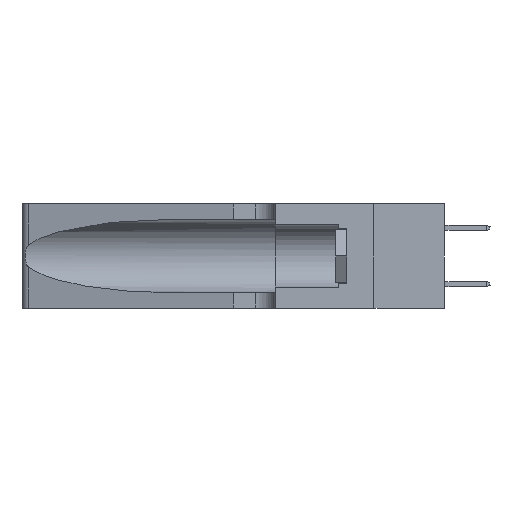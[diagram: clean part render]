
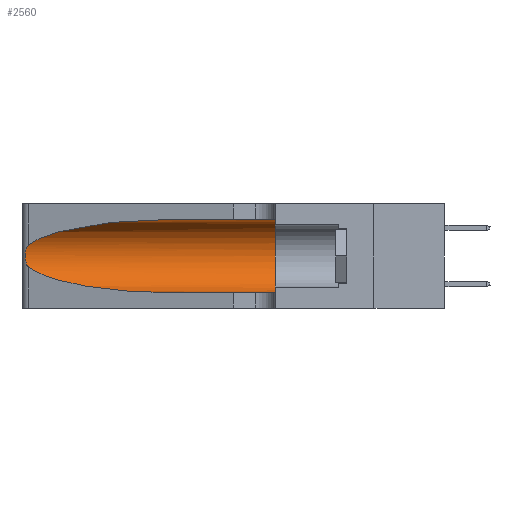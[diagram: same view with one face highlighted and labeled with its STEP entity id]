
A CAD part, left-side view. The second image highlights one B-rep face of the part: STEP entity #2560.
In plain terms, the highlighted cylindrical face has radius 3.308 mm (diameter 6.617 mm), a partial arc.
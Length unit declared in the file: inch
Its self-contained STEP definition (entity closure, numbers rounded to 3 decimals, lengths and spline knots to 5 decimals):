
#1256 = EDGE_CURVE ( 'NONE', #25489, #33092, #20155, .T. ) ;
#1306 = CARTESIAN_POINT ( 'NONE',  ( 0.1305, 0.35, 0.185 ) ) ;
#1328 = DIRECTION ( 'NONE',  ( 0., -1., 0. ) ) ;
#1472 = DIRECTION ( 'NONE',  ( 0., 0., -1. ) ) ;
#2560 = ADVANCED_FACE ( 'NONE', ( #18975 ), #17908, .F. ) ;
#2802 = CARTESIAN_POINT ( 'NONE',  ( 0.25639, 1.23186, 0.15144 ) ) ;
#3285 = VERTEX_POINT ( 'NONE', #24985 ) ;
#3725 = VERTEX_POINT ( 'NONE', #6746 ) ;
#4395 = EDGE_CURVE ( 'NONE', #14317, #3725, #28482, .T. ) ;
#4875 = CARTESIAN_POINT ( 'NONE',  ( 0.2373, 1.15595, 0.28018 ) ) ;
#5112 = ORIENTED_EDGE ( 'NONE', *, *, #26190, .T. ) ;
#5390 = CARTESIAN_POINT ( 'NONE',  ( 0.1305, 0.35, 0.31525 ) ) ;
#5917 = ORIENTED_EDGE ( 'NONE', *, *, #1256, .T. ) ;
#6312 = CARTESIAN_POINT ( 'NONE',  ( 0.25487, 1.22718, 0.14631 ) ) ;
#6466 = EDGE_CURVE ( 'NONE', #3285, #15598, #8846, .T. ) ;
#6746 = CARTESIAN_POINT ( 'NONE',  ( 0.25487, 1.22718, 0.14631 ) ) ;
#8054 = CARTESIAN_POINT ( 'NONE',  ( 0.18966, 0.96281, 0.31525 ) ) ;
#8457 = CIRCLE ( 'NONE', #26831, 0.13025 ) ;
#8846 = LINE ( 'NONE', #23445, #31227 ) ;
#9050 = CARTESIAN_POINT ( 'NONE',  ( 0.26017, 1.23833, 0.17102 ) ) ;
#9382 = EDGE_LOOP ( 'NONE', ( #5112, #15748, #40981, #5917, #18260, #11032 ) ) ;
#9678 = CARTESIAN_POINT ( 'NONE',  ( 0.2373, 1.15595, 0.08982 ) ) ;
#11032 = ORIENTED_EDGE ( 'NONE', *, *, #6466, .F. ) ;
#12369 = CARTESIAN_POINT ( 'NONE',  ( 0.26075, 1.23896, 0.178 ) ) ;
#13435 = CARTESIAN_POINT ( 'NONE',  ( 0.18966, 0.96281, 0.05475 ) ) ;
#14317 = VERTEX_POINT ( 'NONE', #18266 ) ;
#15598 = VERTEX_POINT ( 'NONE', #5390 ) ;
#15748 = ORIENTED_EDGE ( 'NONE', *, *, #4395, .T. ) ;
#15858 = CARTESIAN_POINT ( 'NONE',  ( 0.25555, 1.22994, 0.2215 ) ) ;
#16002 = CARTESIAN_POINT ( 'NONE',  ( 0.25854, 1.2359, 0.20912 ) ) ;
#16900 = EDGE_CURVE ( 'NONE', #3725, #25489, #34334, .T. ) ;
#17908 = CYLINDRICAL_SURFACE ( 'NONE', #33889, 0.13025 ) ;
#17938 = CARTESIAN_POINT ( 'NONE',  ( 0.25487, 1.22718, 0.22369 ) ) ;
#18260 = ORIENTED_EDGE ( 'NONE', *, *, #27391, .F. ) ;
#18266 = CARTESIAN_POINT ( 'NONE',  ( 0.25487, 1.22718, 0.22369 ) ) ;
#18975 = FACE_OUTER_BOUND ( 'NONE', #9382, .T. ) ;
#19218 = CARTESIAN_POINT ( 'NONE',  ( 0.25856, 1.23593, 0.16098 ) ) ;
#19651 = CARTESIAN_POINT ( 'NONE',  ( 0.26075, 1.23896, 0.19203 ) ) ;
#20155 = LINE ( 'NONE', #31226, #35750 ) ;
#21203 = DIRECTION ( 'NONE',  ( 0., -1., 0. ) ) ;
#22607 = CARTESIAN_POINT ( 'NONE',  ( 0.25487, 1.22718, 0.22369 ) ) ;
#22744 = CARTESIAN_POINT ( 'NONE',  ( 0.25789, 1.23486, 0.15765 ) ) ;
#23040 = CARTESIAN_POINT ( 'NONE',  ( 0.26018, 1.23835, 0.19895 ) ) ;
#23445 = CARTESIAN_POINT ( 'NONE',  ( 0.1305, 1.61858, 0.31525 ) ) ;
#24471 = CARTESIAN_POINT ( 'NONE',  ( 0.1305, 1.61858, 0.185 ) ) ;
#24597 = DIRECTION ( 'NONE',  ( 0., 0., 1. ) ) ;
#24985 = CARTESIAN_POINT ( 'NONE',  ( 0.1305, 0.72297, 0.31525 ) ) ;
#25408 = CARTESIAN_POINT ( 'NONE',  ( 0.1305, 0.35, 0.05475 ) ) ;
#25489 = VERTEX_POINT ( 'NONE', #27231 ) ;
#26190 = EDGE_CURVE ( 'NONE', #3285, #14317, #37522, .T. ) ;
#26831 = AXIS2_PLACEMENT_3D ( 'NONE', #1306, #30684, #24597 ) ;
#27231 = CARTESIAN_POINT ( 'NONE',  ( 0.1305, 0.72297, 0.05475 ) ) ;
#27391 = EDGE_CURVE ( 'NONE', #15598, #33092, #8457, .T. ) ;
#28482 = B_SPLINE_CURVE_WITH_KNOTS ( 'NONE', 3,
 ( #22607, #15858, #39569, #39144, #16002, #23040, #19651, #12369, #9050, #19218, #22744, #2802, #42460, #32611 ),
 .UNSPECIFIED., .F., .F.,
 ( 4, 2, 2, 2, 2, 2, 4 ),
 ( 0., 0.00027, 0.00053, 0.00107, 0.0016, 0.00187, 0.00214 ),
 .UNSPECIFIED. ) ;
#30684 = DIRECTION ( 'NONE',  ( 0., 1., 0. ) ) ;
#31226 = CARTESIAN_POINT ( 'NONE',  ( 0.1305, 1.61858, 0.05475 ) ) ;
#31227 = VECTOR ( 'NONE', #40127, 39.37008 ) ;
#32611 = CARTESIAN_POINT ( 'NONE',  ( 0.25487, 1.22718, 0.14631 ) ) ;
#33092 = VERTEX_POINT ( 'NONE', #25408 ) ;
#33889 = AXIS2_PLACEMENT_3D ( 'NONE', #24471, #1328, #1472 ) ;
#34334 =( BOUNDED_CURVE ( )  B_SPLINE_CURVE ( 3, ( #6312, #9678, #13435, #39765 ),
 .UNSPECIFIED., .F., .F. ) 
 B_SPLINE_CURVE_WITH_KNOTS ( ( 4, 4 ),
 ( 3.44316, 4.71239 ),
 .UNSPECIFIED. ) 
 CURVE ( )  GEOMETRIC_REPRESENTATION_ITEM ( )  RATIONAL_B_SPLINE_CURVE ( ( 1., 0.87, 0.87, 1. ) ) 
 REPRESENTATION_ITEM ( '' )  );
#35750 = VECTOR ( 'NONE', #21203, 39.37008 ) ;
#37522 =( BOUNDED_CURVE ( )  B_SPLINE_CURVE ( 3, ( #41474, #8054, #4875, #17938 ),
 .UNSPECIFIED., .F., .F. ) 
 B_SPLINE_CURVE_WITH_KNOTS ( ( 4, 4 ),
 ( 1.5708, 2.84003 ),
 .UNSPECIFIED. ) 
 CURVE ( )  GEOMETRIC_REPRESENTATION_ITEM ( )  RATIONAL_B_SPLINE_CURVE ( ( 1., 0.87, 0.87, 1. ) ) 
 REPRESENTATION_ITEM ( '' )  );
#39144 = CARTESIAN_POINT ( 'NONE',  ( 0.25787, 1.23484, 0.2124 ) ) ;
#39569 = CARTESIAN_POINT ( 'NONE',  ( 0.25639, 1.23184, 0.21858 ) ) ;
#39765 = CARTESIAN_POINT ( 'NONE',  ( 0.1305, 0.72297, 0.05475 ) ) ;
#40127 = DIRECTION ( 'NONE',  ( 0., -1., 0. ) ) ;
#40981 = ORIENTED_EDGE ( 'NONE', *, *, #16900, .T. ) ;
#41474 = CARTESIAN_POINT ( 'NONE',  ( 0.1305, 0.72297, 0.31525 ) ) ;
#42460 = CARTESIAN_POINT ( 'NONE',  ( 0.25555, 1.22993, 0.14849 ) ) ;
